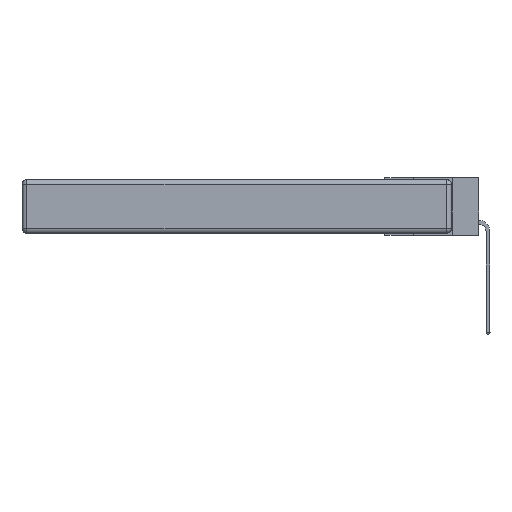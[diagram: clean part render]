
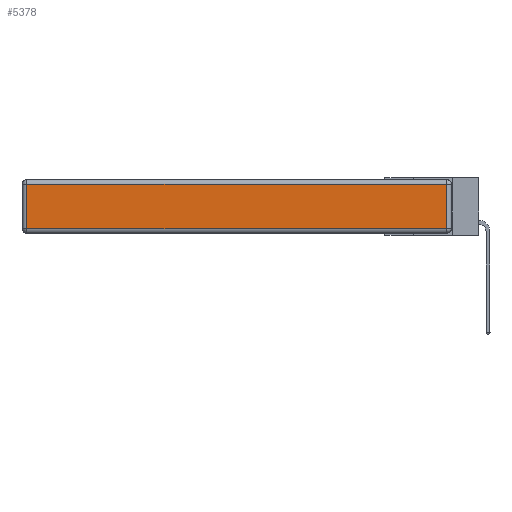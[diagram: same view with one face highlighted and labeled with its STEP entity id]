
A CAD part, left-side view. The second image highlights one B-rep face of the part: STEP entity #5378.
In plain terms, the highlighted planar face has unit normal (-1, 0, 0).
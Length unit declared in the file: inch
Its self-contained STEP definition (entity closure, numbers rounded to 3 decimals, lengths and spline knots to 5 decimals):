
#682 = FACE_OUTER_BOUND ( 'NONE', #20491, .T. ) ;
#868 = CARTESIAN_POINT ( 'NONE',  ( 0., 2.72, -0.03 ) ) ;
#2330 = ORIENTED_EDGE ( 'NONE', *, *, #17110, .T. ) ;
#2379 = VERTEX_POINT ( 'NONE', #11837 ) ;
#2645 = DIRECTION ( 'NONE',  ( 0., 0., 1. ) ) ;
#2937 = DIRECTION ( 'NONE',  ( 0., 0., 1. ) ) ;
#2951 = AXIS2_PLACEMENT_3D ( 'NONE', #16827, #20339, #2937 ) ;
#4084 = LINE ( 'NONE', #19826, #12782 ) ;
#4209 = ORIENTED_EDGE ( 'NONE', *, *, #16470, .T. ) ;
#4782 = VERTEX_POINT ( 'NONE', #868 ) ;
#5378 = ADVANCED_FACE ( 'NONE', ( #682 ), #13159, .T. ) ;
#6454 = VERTEX_POINT ( 'NONE', #15898 ) ;
#6864 = VERTEX_POINT ( 'NONE', #9366 ) ;
#7740 = ORIENTED_EDGE ( 'NONE', *, *, #15788, .T. ) ;
#7851 = CARTESIAN_POINT ( 'NONE',  ( 0., 0.03, -0.343 ) ) ;
#9366 = CARTESIAN_POINT ( 'NONE',  ( 0., 0.03, -0.313 ) ) ;
#11609 = VECTOR ( 'NONE', #18474, 39.37008 ) ;
#11653 = VECTOR ( 'NONE', #2645, 39.37008 ) ;
#11837 = CARTESIAN_POINT ( 'NONE',  ( 0., 2.72, -0.313 ) ) ;
#11877 = DIRECTION ( 'NONE',  ( 0., -1., 0. ) ) ;
#11953 = ORIENTED_EDGE ( 'NONE', *, *, #15648, .T. ) ;
#12782 = VECTOR ( 'NONE', #19689, 39.37008 ) ;
#13125 = CARTESIAN_POINT ( 'NONE',  ( 0., 2.72, -0.343 ) ) ;
#13159 = PLANE ( 'NONE',  #2951 ) ;
#13554 = CARTESIAN_POINT ( 'NONE',  ( 0., 0., -0.313 ) ) ;
#15648 = EDGE_CURVE ( 'NONE', #6454, #4782, #4084, .T. ) ;
#15788 = EDGE_CURVE ( 'NONE', #2379, #6864, #16861, .T. ) ;
#15898 = CARTESIAN_POINT ( 'NONE',  ( 0., 0.03, -0.03 ) ) ;
#16470 = EDGE_CURVE ( 'NONE', #6864, #6454, #19294, .T. ) ;
#16827 = CARTESIAN_POINT ( 'NONE',  ( 0., 0., -0.343 ) ) ;
#16861 = LINE ( 'NONE', #13554, #18249 ) ;
#17110 = EDGE_CURVE ( 'NONE', #4782, #2379, #18990, .T. ) ;
#18249 = VECTOR ( 'NONE', #11877, 39.37008 ) ;
#18474 = DIRECTION ( 'NONE',  ( 0., 0., -1. ) ) ;
#18990 = LINE ( 'NONE', #13125, #11609 ) ;
#19294 = LINE ( 'NONE', #7851, #11653 ) ;
#19689 = DIRECTION ( 'NONE',  ( 0., 1., 0. ) ) ;
#19826 = CARTESIAN_POINT ( 'NONE',  ( 0., 2.75, -0.03 ) ) ;
#20339 = DIRECTION ( 'NONE',  ( -1., 0., 0. ) ) ;
#20491 = EDGE_LOOP ( 'NONE', ( #7740, #4209, #11953, #2330 ) ) ;
